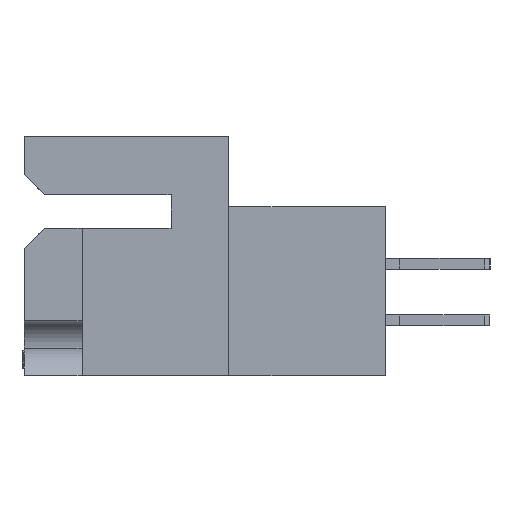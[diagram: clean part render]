
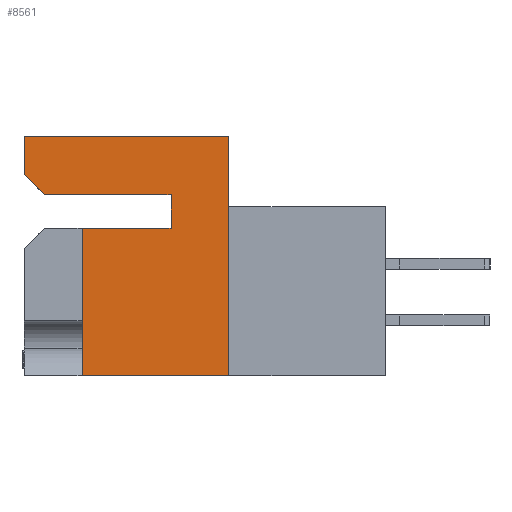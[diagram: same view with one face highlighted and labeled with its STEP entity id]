
A CAD part, left-side view. The second image highlights one B-rep face of the part: STEP entity #8561.
In plain terms, the highlighted planar face has unit normal (-1, 0, 0).
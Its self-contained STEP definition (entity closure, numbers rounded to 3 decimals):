
#887 = CARTESIAN_POINT ( 'NONE',  ( 0., 11.506, -2.159 ) ) ;
#923 = VECTOR ( 'NONE', #9948, 1000. ) ;
#1430 = CARTESIAN_POINT ( 'NONE',  ( 0., 3.251, -3.302 ) ) ;
#1606 = VECTOR ( 'NONE', #36937, 1000. ) ;
#2371 = LINE ( 'NONE', #10504, #923 ) ;
#3007 = VECTOR ( 'NONE', #20770, 1000. ) ;
#3193 = DIRECTION ( 'NONE',  ( 0., 1., 0. ) ) ;
#4443 = LINE ( 'NONE', #18888, #36878 ) ;
#5208 = EDGE_CURVE ( 'NONE', #28124, #34793, #2371, .T. ) ;
#6524 = LINE ( 'NONE', #13598, #30627 ) ;
#7063 = VERTEX_POINT ( 'NONE', #19182 ) ;
#8141 = LINE ( 'NONE', #22042, #40088 ) ;
#8276 = VECTOR ( 'NONE', #23841, 1000. ) ;
#8561 = ADVANCED_FACE ( 'NONE', ( #15779 ), #21354, .F. ) ;
#8613 = EDGE_LOOP ( 'NONE', ( #13350, #39397, #31566, #27895, #8985, #15524, #32505, #37844, #29062 ) ) ;
#8691 = DIRECTION ( 'NONE',  ( 1., 0., 0. ) ) ;
#8985 = ORIENTED_EDGE ( 'NONE', *, *, #16661, .T. ) ;
#9365 = AXIS2_PLACEMENT_3D ( 'NONE', #18471, #8691, #40572 ) ;
#9948 = DIRECTION ( 'NONE',  ( 0., 1., 0. ) ) ;
#10421 = LINE ( 'NONE', #37264, #33541 ) ;
#10446 = EDGE_CURVE ( 'NONE', #18528, #26518, #27946, .T. ) ;
#10504 = CARTESIAN_POINT ( 'NONE',  ( 0., -8.814, -13.487 ) ) ;
#12967 = VERTEX_POINT ( 'NONE', #887 ) ;
#13350 = ORIENTED_EDGE ( 'NONE', *, *, #5208, .F. ) ;
#13598 = CARTESIAN_POINT ( 'NONE',  ( 0., 3.251, -5.182 ) ) ;
#14333 = LINE ( 'NONE', #14849, #3007 ) ;
#14849 = CARTESIAN_POINT ( 'NONE',  ( 0., 0., 0. ) ) ;
#15386 = EDGE_CURVE ( 'NONE', #12967, #18528, #4443, .T. ) ;
#15441 = EDGE_CURVE ( 'NONE', #37471, #35825, #8141, .T. ) ;
#15524 = ORIENTED_EDGE ( 'NONE', *, *, #15441, .F. ) ;
#15779 = FACE_OUTER_BOUND ( 'NONE', #8613, .T. ) ;
#15843 = EDGE_CURVE ( 'NONE', #20788, #37471, #6524, .T. ) ;
#15975 = EDGE_CURVE ( 'NONE', #34793, #7063, #25655, .T. ) ;
#16655 = LINE ( 'NONE', #33850, #8276 ) ;
#16661 = EDGE_CURVE ( 'NONE', #12967, #35825, #10421, .T. ) ;
#18471 = CARTESIAN_POINT ( 'NONE',  ( 0., 0., 0. ) ) ;
#18528 = VERTEX_POINT ( 'NONE', #37435 ) ;
#18888 = CARTESIAN_POINT ( 'NONE',  ( 0., 11.506, -13.487 ) ) ;
#19182 = CARTESIAN_POINT ( 'NONE',  ( 0., 8.255, -5.182 ) ) ;
#19262 = CARTESIAN_POINT ( 'NONE',  ( 0., 8.255, -13.487 ) ) ;
#20770 = DIRECTION ( 'NONE',  ( 0., 0., -1. ) ) ;
#20788 = VERTEX_POINT ( 'NONE', #23242 ) ;
#21354 = PLANE ( 'NONE',  #9365 ) ;
#22042 = CARTESIAN_POINT ( 'NONE',  ( 0., 0., -3.302 ) ) ;
#22280 = DIRECTION ( 'NONE',  ( 0., -1., 0. ) ) ;
#23242 = CARTESIAN_POINT ( 'NONE',  ( 0., 3.251, -5.182 ) ) ;
#23841 = DIRECTION ( 'NONE',  ( 0., -1., 0. ) ) ;
#24587 = CARTESIAN_POINT ( 'NONE',  ( 0., 8.255, -5.182 ) ) ;
#25655 = LINE ( 'NONE', #24587, #1606 ) ;
#25664 = DIRECTION ( 'NONE',  ( 0., 0., 1. ) ) ;
#26518 = VERTEX_POINT ( 'NONE', #38359 ) ;
#26781 = EDGE_CURVE ( 'NONE', #26518, #28124, #14333, .T. ) ;
#27895 = ORIENTED_EDGE ( 'NONE', *, *, #15386, .F. ) ;
#27946 = LINE ( 'NONE', #37929, #28457 ) ;
#28124 = VERTEX_POINT ( 'NONE', #33446 ) ;
#28457 = VECTOR ( 'NONE', #22280, 1000. ) ;
#29062 = ORIENTED_EDGE ( 'NONE', *, *, #15975, .F. ) ;
#30627 = VECTOR ( 'NONE', #25664, 1000. ) ;
#30770 = EDGE_CURVE ( 'NONE', #7063, #20788, #16655, .T. ) ;
#31087 = DIRECTION ( 'NONE',  ( 0., 0., 1. ) ) ;
#31566 = ORIENTED_EDGE ( 'NONE', *, *, #10446, .F. ) ;
#31941 = CARTESIAN_POINT ( 'NONE',  ( 0., 10.363, -3.302 ) ) ;
#32505 = ORIENTED_EDGE ( 'NONE', *, *, #15843, .F. ) ;
#33446 = CARTESIAN_POINT ( 'NONE',  ( 0., 0., -13.487 ) ) ;
#33541 = VECTOR ( 'NONE', #33861, 1000. ) ;
#33850 = CARTESIAN_POINT ( 'NONE',  ( 0., 0., -5.182 ) ) ;
#33861 = DIRECTION ( 'NONE',  ( 0., -0.707, -0.707 ) ) ;
#34793 = VERTEX_POINT ( 'NONE', #19262 ) ;
#35825 = VERTEX_POINT ( 'NONE', #31941 ) ;
#36878 = VECTOR ( 'NONE', #31087, 1000. ) ;
#36937 = DIRECTION ( 'NONE',  ( 0., 0., 1. ) ) ;
#37264 = CARTESIAN_POINT ( 'NONE',  ( 0., 10.363, -3.302 ) ) ;
#37435 = CARTESIAN_POINT ( 'NONE',  ( 0., 11.506, 0. ) ) ;
#37471 = VERTEX_POINT ( 'NONE', #1430 ) ;
#37844 = ORIENTED_EDGE ( 'NONE', *, *, #30770, .F. ) ;
#37929 = CARTESIAN_POINT ( 'NONE',  ( 0., 11.506, 0. ) ) ;
#38359 = CARTESIAN_POINT ( 'NONE',  ( 0., 0., 0. ) ) ;
#39397 = ORIENTED_EDGE ( 'NONE', *, *, #26781, .F. ) ;
#40088 = VECTOR ( 'NONE', #3193, 1000. ) ;
#40572 = DIRECTION ( 'NONE',  ( 0., 0., -1. ) ) ;
